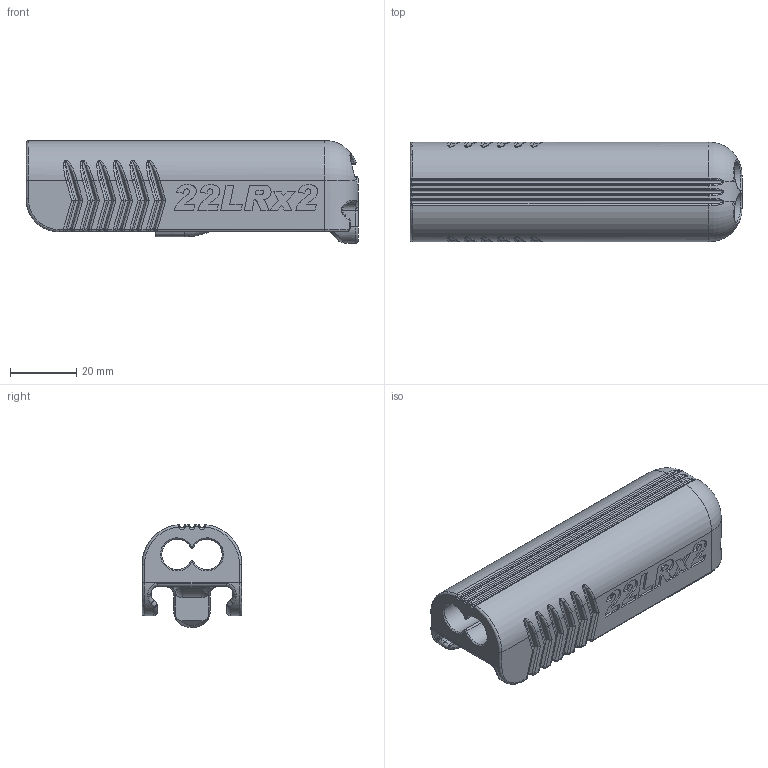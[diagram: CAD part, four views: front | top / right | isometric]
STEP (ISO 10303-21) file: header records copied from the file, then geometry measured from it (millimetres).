
FILE_DESCRIPTION(('FreeCAD Model'),'2;1');
FILE_NAME('Open CASCADE Shape Model','2022-12-07T11:22:52',('Author'),( ''),'Open CASCADE STEP processor 7.6','FreeCAD','Unknown');
FILE_SCHEMA(('AUTOMOTIVE_DESIGN { 1 0 10303 214 1 1 1 1 }'));
Products named in the file (1): Slide x2
Bounding box: 100 x 30 x 31 mm (x, y, z)
Volume: 45844.7 mm3; surface area: 19442.1 mm2
Topology: 1 solids, 1 shells, 706 faces, 1784 edges, 1094 vertices
Faces by surface type: bspline 196, plane 193, cylinder 167, extrusion 116, torus 25, revolution 6, cone 3
Full cylindrical faces by diameter (mm): 2 x1
Entity records: 87628 total; most frequent: CARTESIAN_POINT 57167, DIRECTION 3929, ORIENTED_EDGE 3568, PCURVE 3568, DEFINITIONAL_REPRESENTATION 3568, VECTOR 2742, LINE 2626, B_SPLINE_CURVE_WITH_KNOTS 2126
